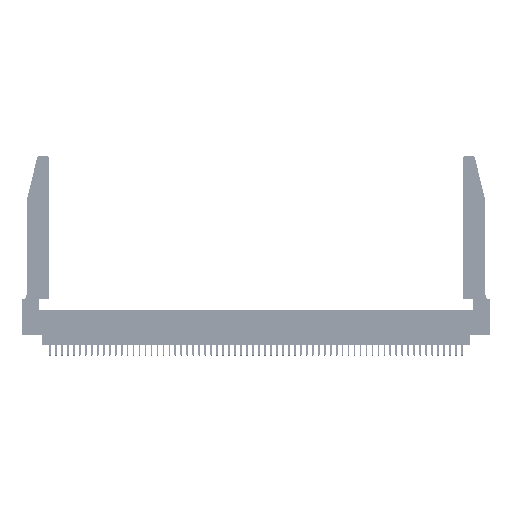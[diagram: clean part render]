
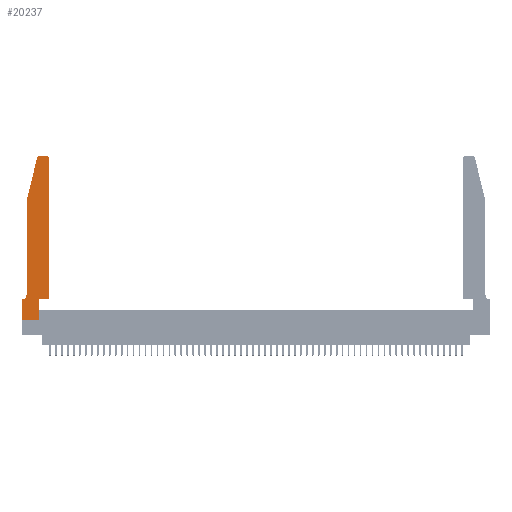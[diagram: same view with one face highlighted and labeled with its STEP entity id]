
A CAD part, top view. The second image highlights one B-rep face of the part: STEP entity #20237.
In plain terms, the highlighted planar face has unit normal (0, 0, 1).
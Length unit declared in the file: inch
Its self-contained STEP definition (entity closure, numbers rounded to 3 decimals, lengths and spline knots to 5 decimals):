
#1199 = CIRCLE ( 'NONE', #45706, 0.03 ) ;
#2175 = CARTESIAN_POINT ( 'NONE',  ( 0.4505, 0.35, 0.37 ) ) ;
#2332 = LINE ( 'NONE', #10767, #32829 ) ;
#2706 = DIRECTION ( 'NONE',  ( -1., 0., 0. ) ) ;
#3283 = VERTEX_POINT ( 'NONE', #54831 ) ;
#3393 = LINE ( 'NONE', #46897, #26429 ) ;
#3549 = DIRECTION ( 'NONE',  ( 1., 0., 0. ) ) ;
#3654 = EDGE_CURVE ( 'NONE', #6387, #33385, #1199, .T. ) ;
#3779 = ORIENTED_EDGE ( 'NONE', *, *, #37839, .T. ) ;
#4990 = DIRECTION ( 'NONE',  ( -1., 0., 0. ) ) ;
#6053 = LINE ( 'NONE', #16520, #39229 ) ;
#6150 = VERTEX_POINT ( 'NONE', #10474 ) ;
#6387 = VERTEX_POINT ( 'NONE', #23661 ) ;
#7818 = CARTESIAN_POINT ( 'NONE',  ( 0.2865, 0.35, 0.37 ) ) ;
#8181 = EDGE_CURVE ( 'NONE', #8340, #17639, #15557, .T. ) ;
#8340 = VERTEX_POINT ( 'NONE', #10735 ) ;
#8514 = AXIS2_PLACEMENT_3D ( 'NONE', #9989, #40295, #14323 ) ;
#8672 = CIRCLE ( 'NONE', #8514, 0.07 ) ;
#8759 = CARTESIAN_POINT ( 'NONE',  ( 0.2865, 0., 0.37 ) ) ;
#8840 = VECTOR ( 'NONE', #11169, 39.37008 ) ;
#9989 = CARTESIAN_POINT ( 'NONE',  ( 0.0055, 0.42, 0.37 ) ) ;
#10201 = CARTESIAN_POINT ( 'NONE',  ( 0.0755, 2., 0.37 ) ) ;
#10474 = CARTESIAN_POINT ( 'NONE',  ( 0., 0.35, 0.37 ) ) ;
#10735 = CARTESIAN_POINT ( 'NONE',  ( 0.25487, 2.72718, 0.37 ) ) ;
#10740 = EDGE_CURVE ( 'NONE', #44918, #43971, #8672, .T. ) ;
#10767 = CARTESIAN_POINT ( 'NONE',  ( 0.0755, 2., 0.37 ) ) ;
#10963 = VECTOR ( 'NONE', #2706, 39.37008 ) ;
#11169 = DIRECTION ( 'NONE',  ( 1., 0., 0. ) ) ;
#11709 = AXIS2_PLACEMENT_3D ( 'NONE', #16406, #46727, #20768 ) ;
#11846 = ORIENTED_EDGE ( 'NONE', *, *, #27445, .T. ) ;
#12514 = DIRECTION ( 'NONE',  ( 0., -1., 0. ) ) ;
#13262 = ORIENTED_EDGE ( 'NONE', *, *, #24104, .T. ) ;
#13286 = CARTESIAN_POINT ( 'NONE',  ( 0.2865, 0.35, 0.37 ) ) ;
#13376 = CARTESIAN_POINT ( 'NONE',  ( 0.0755, 2., 0.37 ) ) ;
#13491 = DIRECTION ( 'NONE',  ( 0., 1., 0. ) ) ;
#13669 = CARTESIAN_POINT ( 'NONE',  ( 0.4505, 0.35, 0.37 ) ) ;
#14321 = CARTESIAN_POINT ( 'NONE',  ( 0.4205, 2.72, 0.37 ) ) ;
#14323 = DIRECTION ( 'NONE',  ( -1., 0., 0. ) ) ;
#15557 = LINE ( 'NONE', #13376, #47445 ) ;
#16406 = CARTESIAN_POINT ( 'NONE',  ( 0.284, 2.72, 0.37 ) ) ;
#16520 = CARTESIAN_POINT ( 'NONE',  ( 0., 0., 0.37 ) ) ;
#16551 = VECTOR ( 'NONE', #13491, 39.37008 ) ;
#16765 = VERTEX_POINT ( 'NONE', #13669 ) ;
#17302 = ORIENTED_EDGE ( 'NONE', *, *, #10740, .T. ) ;
#17432 = CIRCLE ( 'NONE', #11709, 0.03 ) ;
#17639 = VERTEX_POINT ( 'NONE', #10201 ) ;
#17879 = EDGE_CURVE ( 'NONE', #3283, #8340, #17432, .T. ) ;
#18693 = DIRECTION ( 'NONE',  ( 1., 0., 0. ) ) ;
#20237 = ADVANCED_FACE ( 'NONE', ( #48478 ), #50678, .T. ) ;
#20281 = CARTESIAN_POINT ( 'NONE',  ( 0., 0., 0.37 ) ) ;
#20750 = EDGE_CURVE ( 'NONE', #17639, #44918, #2332, .T. ) ;
#20768 = DIRECTION ( 'NONE',  ( 1., 0., 0. ) ) ;
#21273 = LINE ( 'NONE', #22210, #54566 ) ;
#22210 = CARTESIAN_POINT ( 'NONE',  ( 0.2605, 2.75, 0.37 ) ) ;
#22236 = VECTOR ( 'NONE', #32477, 39.37008 ) ;
#23661 = CARTESIAN_POINT ( 'NONE',  ( 0.4505, 2.72, 0.37 ) ) ;
#24104 = EDGE_CURVE ( 'NONE', #33385, #3283, #21273, .T. ) ;
#24680 = CARTESIAN_POINT ( 'NONE',  ( 0., 0.35, 0.37 ) ) ;
#24838 = ORIENTED_EDGE ( 'NONE', *, *, #8181, .T. ) ;
#26429 = VECTOR ( 'NONE', #3549, 39.37008 ) ;
#27445 = EDGE_CURVE ( 'NONE', #51634, #47900, #3393, .T. ) ;
#28618 = CARTESIAN_POINT ( 'NONE',  ( 0.0755, 0.35, 0.37 ) ) ;
#28852 = ORIENTED_EDGE ( 'NONE', *, *, #42662, .T. ) ;
#29034 = DIRECTION ( 'NONE',  ( 1., 0., 0. ) ) ;
#29193 = LINE ( 'NONE', #50283, #8840 ) ;
#30862 = DIRECTION ( 'NONE',  ( -0.239, -0.971, 0. ) ) ;
#30888 = ORIENTED_EDGE ( 'NONE', *, *, #17879, .T. ) ;
#32477 = DIRECTION ( 'NONE',  ( 0., 1., 0. ) ) ;
#32614 = EDGE_CURVE ( 'NONE', #43971, #6150, #55808, .T. ) ;
#32829 = VECTOR ( 'NONE', #45452, 39.37008 ) ;
#33385 = VERTEX_POINT ( 'NONE', #54573 ) ;
#36043 = CARTESIAN_POINT ( 'NONE',  ( 0.0755, 0.42, 0.37 ) ) ;
#37839 = EDGE_CURVE ( 'NONE', #16765, #6387, #51419, .T. ) ;
#39229 = VECTOR ( 'NONE', #12514, 39.37008 ) ;
#39693 = EDGE_CURVE ( 'NONE', #47900, #42604, #40974, .T. ) ;
#40295 = DIRECTION ( 'NONE',  ( 0., 0., -1. ) ) ;
#40974 = LINE ( 'NONE', #13286, #16551 ) ;
#42604 = VERTEX_POINT ( 'NONE', #7818 ) ;
#42662 = EDGE_CURVE ( 'NONE', #6150, #51634, #6053, .T. ) ;
#43971 = VERTEX_POINT ( 'NONE', #55520 ) ;
#44398 = ORIENTED_EDGE ( 'NONE', *, *, #3654, .T. ) ;
#44651 = DIRECTION ( 'NONE',  ( 0., 0., 1. ) ) ;
#44918 = VERTEX_POINT ( 'NONE', #36043 ) ;
#45452 = DIRECTION ( 'NONE',  ( 0., -1., 0. ) ) ;
#45693 = ORIENTED_EDGE ( 'NONE', *, *, #48260, .T. ) ;
#45706 = AXIS2_PLACEMENT_3D ( 'NONE', #14321, #44651, #18693 ) ;
#45935 = AXIS2_PLACEMENT_3D ( 'NONE', #24680, #55060, #29034 ) ;
#46727 = DIRECTION ( 'NONE',  ( 0., 0., 1. ) ) ;
#46897 = CARTESIAN_POINT ( 'NONE',  ( 0., 0., 0.37 ) ) ;
#47445 = VECTOR ( 'NONE', #30862, 39.37008 ) ;
#47769 = EDGE_LOOP ( 'NONE', ( #13262, #30888, #24838, #54033, #17302, #49178, #28852, #11846, #56022, #45693, #3779, #44398 ) ) ;
#47900 = VERTEX_POINT ( 'NONE', #8759 ) ;
#48260 = EDGE_CURVE ( 'NONE', #42604, #16765, #29193, .T. ) ;
#48478 = FACE_OUTER_BOUND ( 'NONE', #47769, .T. ) ;
#49178 = ORIENTED_EDGE ( 'NONE', *, *, #32614, .T. ) ;
#50283 = CARTESIAN_POINT ( 'NONE',  ( 0.4505, 0.35, 0.37 ) ) ;
#50678 = PLANE ( 'NONE',  #45935 ) ;
#51419 = LINE ( 'NONE', #2175, #22236 ) ;
#51634 = VERTEX_POINT ( 'NONE', #20281 ) ;
#54033 = ORIENTED_EDGE ( 'NONE', *, *, #20750, .T. ) ;
#54566 = VECTOR ( 'NONE', #4990, 39.37008 ) ;
#54573 = CARTESIAN_POINT ( 'NONE',  ( 0.4205, 2.75, 0.37 ) ) ;
#54831 = CARTESIAN_POINT ( 'NONE',  ( 0.284, 2.75, 0.37 ) ) ;
#55060 = DIRECTION ( 'NONE',  ( 0., 0., 1. ) ) ;
#55520 = CARTESIAN_POINT ( 'NONE',  ( 0.0055, 0.35, 0.37 ) ) ;
#55808 = LINE ( 'NONE', #28618, #10963 ) ;
#56022 = ORIENTED_EDGE ( 'NONE', *, *, #39693, .T. ) ;
